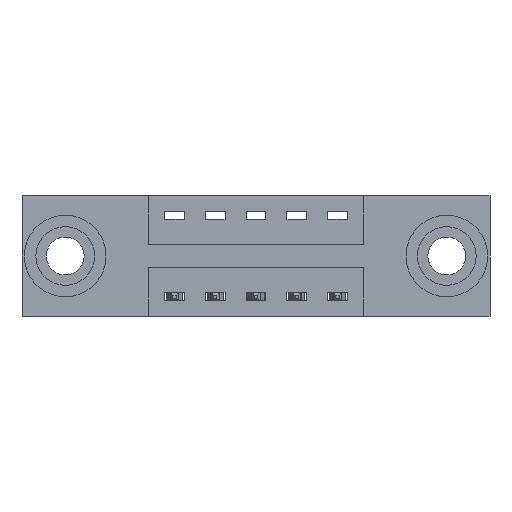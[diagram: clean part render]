
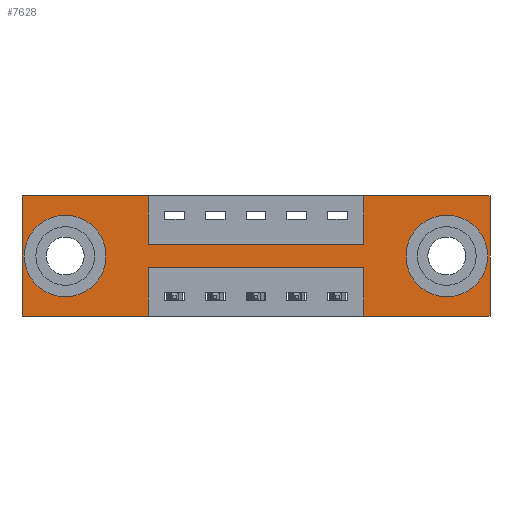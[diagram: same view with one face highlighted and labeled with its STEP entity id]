
A CAD part, front view. The second image highlights one B-rep face of the part: STEP entity #7628.
In plain terms, the highlighted planar face has unit normal (0, -1, 0).
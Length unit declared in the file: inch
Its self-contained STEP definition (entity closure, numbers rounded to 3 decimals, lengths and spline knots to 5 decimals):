
#78 = CARTESIAN_POINT ( 'NONE',  ( 0.3875, 0., -0.15 ) ) ;
#113 = VECTOR ( 'NONE', #7905, 39.37008 ) ;
#165 = LINE ( 'NONE', #5820, #3750 ) ;
#301 = CARTESIAN_POINT ( 'NONE',  ( 1.3025, 0., -0.263 ) ) ;
#403 = VERTEX_POINT ( 'NONE', #5806 ) ;
#553 = EDGE_LOOP ( 'NONE', ( #5614, #8139, #4906, #5742, #3982, #1761, #1540, #3138, #2716, #7589, #6655, #5532 ) ) ;
#571 = AXIS2_PLACEMENT_3D ( 'NONE', #864, #5670, #1644 ) ;
#606 = CARTESIAN_POINT ( 'NONE',  ( 0.3875, 0., -0.22 ) ) ;
#631 = DIRECTION ( 'NONE',  ( 0., 0., 1. ) ) ;
#721 = CARTESIAN_POINT ( 'NONE',  ( 1.435, 0., 0. ) ) ;
#864 = CARTESIAN_POINT ( 'NONE',  ( 0.1325, 0., -0.185 ) ) ;
#990 = VECTOR ( 'NONE', #7337, 39.37008 ) ;
#1000 = VERTEX_POINT ( 'NONE', #6982 ) ;
#1084 = CARTESIAN_POINT ( 'NONE',  ( 0.3875, 0., 0. ) ) ;
#1138 = LINE ( 'NONE', #1374, #2569 ) ;
#1337 = FACE_BOUND ( 'NONE', #3338, .T. ) ;
#1374 = CARTESIAN_POINT ( 'NONE',  ( 0., 0., 0. ) ) ;
#1434 = CARTESIAN_POINT ( 'NONE',  ( 0., 0., 0. ) ) ;
#1540 = ORIENTED_EDGE ( 'NONE', *, *, #4046, .F. ) ;
#1581 = EDGE_CURVE ( 'NONE', #403, #3817, #8474, .T. ) ;
#1644 = DIRECTION ( 'NONE',  ( 0., 0., 1. ) ) ;
#1700 = VERTEX_POINT ( 'NONE', #301 ) ;
#1734 = EDGE_LOOP ( 'NONE', ( #4576, #3655 ) ) ;
#1761 = ORIENTED_EDGE ( 'NONE', *, *, #4676, .F. ) ;
#1858 = CARTESIAN_POINT ( 'NONE',  ( 1.3025, 0., -0.185 ) ) ;
#1894 = CARTESIAN_POINT ( 'NONE',  ( 1.435, 0., -0.37 ) ) ;
#1955 = LINE ( 'NONE', #3192, #7065 ) ;
#1998 = VECTOR ( 'NONE', #2137, 39.37008 ) ;
#2004 = DIRECTION ( 'NONE',  ( 0., 1., 0. ) ) ;
#2011 = VERTEX_POINT ( 'NONE', #1894 ) ;
#2031 = PLANE ( 'NONE',  #3904 ) ;
#2036 = AXIS2_PLACEMENT_3D ( 'NONE', #6001, #2004, #6669 ) ;
#2137 = DIRECTION ( 'NONE',  ( 0., 0., -1. ) ) ;
#2182 = DIRECTION ( 'NONE',  ( 0., 0., -1. ) ) ;
#2263 = VERTEX_POINT ( 'NONE', #8370 ) ;
#2533 = DIRECTION ( 'NONE',  ( 0., 0., -1. ) ) ;
#2569 = VECTOR ( 'NONE', #5409, 39.37008 ) ;
#2642 = LINE ( 'NONE', #6805, #1998 ) ;
#2686 = CARTESIAN_POINT ( 'NONE',  ( 1.0475, 0., -0.22 ) ) ;
#2716 = ORIENTED_EDGE ( 'NONE', *, *, #7105, .F. ) ;
#2718 = DIRECTION ( 'NONE',  ( 0., 0., -1. ) ) ;
#2738 = VECTOR ( 'NONE', #2182, 39.37008 ) ;
#2888 = LINE ( 'NONE', #5336, #990 ) ;
#3137 = VERTEX_POINT ( 'NONE', #1084 ) ;
#3138 = ORIENTED_EDGE ( 'NONE', *, *, #6434, .F. ) ;
#3192 = CARTESIAN_POINT ( 'NONE',  ( 0.3875, 0., -0.22 ) ) ;
#3296 = VERTEX_POINT ( 'NONE', #5308 ) ;
#3338 = EDGE_LOOP ( 'NONE', ( #8335, #5710 ) ) ;
#3427 = CARTESIAN_POINT ( 'NONE',  ( 1.0475, 0., 0. ) ) ;
#3655 = ORIENTED_EDGE ( 'NONE', *, *, #8362, .T. ) ;
#3695 = EDGE_CURVE ( 'NONE', #6564, #403, #6342, .T. ) ;
#3732 = CARTESIAN_POINT ( 'NONE',  ( 1.3025, 0., -0.107 ) ) ;
#3733 = VECTOR ( 'NONE', #631, 39.37008 ) ;
#3743 = DIRECTION ( 'NONE',  ( 0., 0., -1. ) ) ;
#3750 = VECTOR ( 'NONE', #3806, 39.37008 ) ;
#3773 = CARTESIAN_POINT ( 'NONE',  ( 1.3025, 0., -0.185 ) ) ;
#3797 = EDGE_CURVE ( 'NONE', #2011, #5244, #165, .T. ) ;
#3806 = DIRECTION ( 'NONE',  ( -1., 0., 0. ) ) ;
#3813 = EDGE_CURVE ( 'NONE', #5812, #6564, #1955, .T. ) ;
#3817 = VERTEX_POINT ( 'NONE', #8423 ) ;
#3836 = AXIS2_PLACEMENT_3D ( 'NONE', #1858, #6531, #2533 ) ;
#3904 = AXIS2_PLACEMENT_3D ( 'NONE', #8610, #6704, #2718 ) ;
#3982 = ORIENTED_EDGE ( 'NONE', *, *, #8590, .F. ) ;
#4046 = EDGE_CURVE ( 'NONE', #7223, #5581, #7158, .T. ) ;
#4096 = DIRECTION ( 'NONE',  ( 0., 0., 1. ) ) ;
#4222 = VECTOR ( 'NONE', #4696, 39.37008 ) ;
#4348 = VERTEX_POINT ( 'NONE', #3732 ) ;
#4393 = CARTESIAN_POINT ( 'NONE',  ( 1.0475, 0., 0. ) ) ;
#4427 = CIRCLE ( 'NONE', #2036, 0.078 ) ;
#4443 = DIRECTION ( 'NONE',  ( 0., 0., -1. ) ) ;
#4547 = DIRECTION ( 'NONE',  ( -1., 0., 0. ) ) ;
#4576 = ORIENTED_EDGE ( 'NONE', *, *, #4929, .T. ) ;
#4600 = VECTOR ( 'NONE', #3743, 39.37008 ) ;
#4673 = CIRCLE ( 'NONE', #3836, 0.078 ) ;
#4676 = EDGE_CURVE ( 'NONE', #5581, #3296, #1138, .T. ) ;
#4696 = DIRECTION ( 'NONE',  ( 1., 0., 0. ) ) ;
#4747 = EDGE_CURVE ( 'NONE', #3817, #2263, #5501, .T. ) ;
#4906 = ORIENTED_EDGE ( 'NONE', *, *, #5250, .F. ) ;
#4929 = EDGE_CURVE ( 'NONE', #5169, #1000, #5803, .T. ) ;
#4940 = LINE ( 'NONE', #721, #2738 ) ;
#5025 = VECTOR ( 'NONE', #6624, 39.37008 ) ;
#5048 = CARTESIAN_POINT ( 'NONE',  ( 0.3875, 0., -0.37 ) ) ;
#5169 = VERTEX_POINT ( 'NONE', #7888 ) ;
#5244 = VERTEX_POINT ( 'NONE', #7304 ) ;
#5250 = EDGE_CURVE ( 'NONE', #5244, #5812, #2888, .T. ) ;
#5289 = CARTESIAN_POINT ( 'NONE',  ( 0.3875, 0., -0.15 ) ) ;
#5308 = CARTESIAN_POINT ( 'NONE',  ( 1.435, 0., 0. ) ) ;
#5336 = CARTESIAN_POINT ( 'NONE',  ( 1.0475, 0., -0.37 ) ) ;
#5403 = VECTOR ( 'NONE', #4096, 39.37008 ) ;
#5409 = DIRECTION ( 'NONE',  ( 1., 0., 0. ) ) ;
#5501 = LINE ( 'NONE', #1434, #3733 ) ;
#5532 = ORIENTED_EDGE ( 'NONE', *, *, #1581, .F. ) ;
#5581 = VERTEX_POINT ( 'NONE', #4393 ) ;
#5614 = ORIENTED_EDGE ( 'NONE', *, *, #3695, .F. ) ;
#5670 = DIRECTION ( 'NONE',  ( 0., 1., 0. ) ) ;
#5695 = EDGE_CURVE ( 'NONE', #4348, #1700, #4673, .T. ) ;
#5710 = ORIENTED_EDGE ( 'NONE', *, *, #7980, .T. ) ;
#5742 = ORIENTED_EDGE ( 'NONE', *, *, #3797, .F. ) ;
#5803 = CIRCLE ( 'NONE', #571, 0.078 ) ;
#5806 = CARTESIAN_POINT ( 'NONE',  ( 0.3875, 0., -0.37 ) ) ;
#5812 = VERTEX_POINT ( 'NONE', #2686 ) ;
#5820 = CARTESIAN_POINT ( 'NONE',  ( 0., 0., -0.37 ) ) ;
#5956 = LINE ( 'NONE', #8115, #4222 ) ;
#6001 = CARTESIAN_POINT ( 'NONE',  ( 0.1325, 0., -0.185 ) ) ;
#6342 = LINE ( 'NONE', #5048, #4600 ) ;
#6398 = AXIS2_PLACEMENT_3D ( 'NONE', #3773, #8329, #4443 ) ;
#6434 = EDGE_CURVE ( 'NONE', #8714, #7223, #7435, .T. ) ;
#6531 = DIRECTION ( 'NONE',  ( 0., 1., 0. ) ) ;
#6564 = VERTEX_POINT ( 'NONE', #606 ) ;
#6624 = DIRECTION ( 'NONE',  ( -1., 0., 0. ) ) ;
#6655 = ORIENTED_EDGE ( 'NONE', *, *, #4747, .F. ) ;
#6669 = DIRECTION ( 'NONE',  ( 0., 0., 1. ) ) ;
#6704 = DIRECTION ( 'NONE',  ( 0., -1., 0. ) ) ;
#6805 = CARTESIAN_POINT ( 'NONE',  ( 0.3875, 0., 0. ) ) ;
#6916 = FACE_BOUND ( 'NONE', #1734, .T. ) ;
#6982 = CARTESIAN_POINT ( 'NONE',  ( 0.1325, 0., -0.263 ) ) ;
#7000 = CARTESIAN_POINT ( 'NONE',  ( 0., 0., -0.37 ) ) ;
#7065 = VECTOR ( 'NONE', #4547, 39.37008 ) ;
#7105 = EDGE_CURVE ( 'NONE', #3137, #8714, #2642, .T. ) ;
#7158 = LINE ( 'NONE', #3427, #5403 ) ;
#7223 = VERTEX_POINT ( 'NONE', #8179 ) ;
#7304 = CARTESIAN_POINT ( 'NONE',  ( 1.0475, 0., -0.37 ) ) ;
#7337 = DIRECTION ( 'NONE',  ( 0., 0., 1. ) ) ;
#7435 = LINE ( 'NONE', #5289, #113 ) ;
#7589 = ORIENTED_EDGE ( 'NONE', *, *, #8374, .F. ) ;
#7628 = ADVANCED_FACE ( 'NONE', ( #1337, #6916, #7692 ), #2031, .T. ) ;
#7692 = FACE_OUTER_BOUND ( 'NONE', #553, .T. ) ;
#7888 = CARTESIAN_POINT ( 'NONE',  ( 0.1325, 0., -0.107 ) ) ;
#7905 = DIRECTION ( 'NONE',  ( 1., 0., 0. ) ) ;
#7980 = EDGE_CURVE ( 'NONE', #1700, #4348, #8105, .T. ) ;
#8105 = CIRCLE ( 'NONE', #6398, 0.078 ) ;
#8115 = CARTESIAN_POINT ( 'NONE',  ( 0., 0., 0. ) ) ;
#8139 = ORIENTED_EDGE ( 'NONE', *, *, #3813, .F. ) ;
#8179 = CARTESIAN_POINT ( 'NONE',  ( 1.0475, 0., -0.15 ) ) ;
#8329 = DIRECTION ( 'NONE',  ( 0., 1., 0. ) ) ;
#8335 = ORIENTED_EDGE ( 'NONE', *, *, #5695, .T. ) ;
#8362 = EDGE_CURVE ( 'NONE', #1000, #5169, #4427, .T. ) ;
#8370 = CARTESIAN_POINT ( 'NONE',  ( 0., 0., 0. ) ) ;
#8374 = EDGE_CURVE ( 'NONE', #2263, #3137, #5956, .T. ) ;
#8423 = CARTESIAN_POINT ( 'NONE',  ( 0., 0., -0.37 ) ) ;
#8474 = LINE ( 'NONE', #7000, #5025 ) ;
#8590 = EDGE_CURVE ( 'NONE', #3296, #2011, #4940, .T. ) ;
#8610 = CARTESIAN_POINT ( 'NONE',  ( 0., 0., -0.37 ) ) ;
#8714 = VERTEX_POINT ( 'NONE', #78 ) ;
